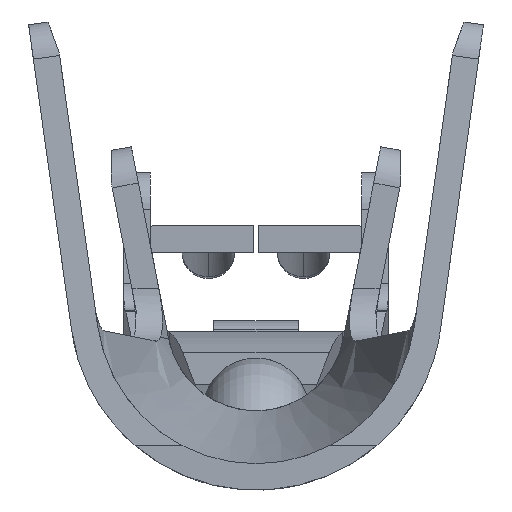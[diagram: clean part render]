
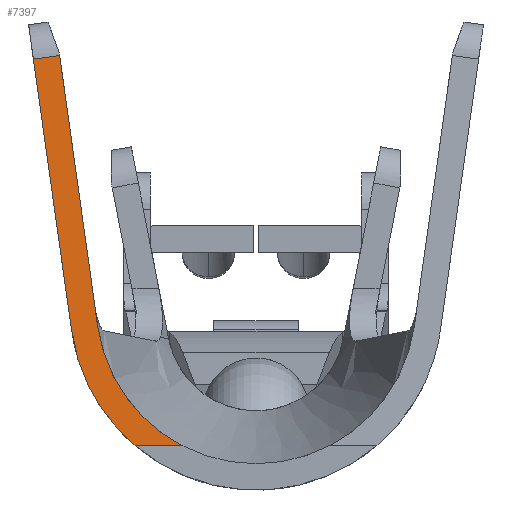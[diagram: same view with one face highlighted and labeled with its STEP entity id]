
A CAD part, front view. The second image highlights one B-rep face of the part: STEP entity #7397.
In plain terms, the highlighted planar face has unit normal (0, -0.998, 0.062).
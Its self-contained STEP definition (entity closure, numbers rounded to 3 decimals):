
#13 = VECTOR ( 'NONE', #1316, 1000. ) ;
#239 = DIRECTION ( 'NONE',  ( 0., -0.062, -0.998 ) ) ;
#319 = EDGE_CURVE ( 'NONE', #6120, #3955, #1105, .T. ) ;
#474 = CARTESIAN_POINT ( 'NONE',  ( -0.93, -4.743, -2.258 ) ) ;
#768 = VERTEX_POINT ( 'NONE', #2035 ) ;
#892 = ORIENTED_EDGE ( 'NONE', *, *, #319, .F. ) ;
#995 = VECTOR ( 'NONE', #4025, 1000. ) ;
#1105 = LINE ( 'NONE', #3718, #8045 ) ;
#1187 = LINE ( 'NONE', #8018, #995 ) ;
#1316 = DIRECTION ( 'NONE',  ( 0.99, 0.009, 0.139 ) ) ;
#1602 = VERTEX_POINT ( 'NONE', #4962 ) ;
#1620 = AXIS2_PLACEMENT_3D ( 'NONE', #6358, #3668, #239 ) ;
#1821 = CARTESIAN_POINT ( 'NONE',  ( -1.275, -4.723, -1.938 ) ) ;
#1880 = EDGE_CURVE ( 'NONE', #1602, #8000, #2816, .T. ) ;
#2035 = CARTESIAN_POINT ( 'NONE',  ( -1.497, -4.68, -1.248 ) ) ;
#2176 = PLANE ( 'NONE',  #1620 ) ;
#2337 = EDGE_CURVE ( 'NONE', #1602, #7081, #8230, .T. ) ;
#2407 = CARTESIAN_POINT ( 'NONE',  ( -1.857, -4.52, 1.31 ) ) ;
#2603 = CARTESIAN_POINT ( 'NONE',  ( -1.144, -4.75, -2.378 ) ) ;
#2770 = CARTESIAN_POINT ( 'NONE',  ( -2.104, -4.522, 1.275 ) ) ;
#2798 = ORIENTED_EDGE ( 'NONE', *, *, #5814, .F. ) ;
#2816 = LINE ( 'NONE', #2770, #4200 ) ;
#2915 = ORIENTED_EDGE ( 'NONE', *, *, #1880, .T. ) ;
#3623 = FACE_OUTER_BOUND ( 'NONE', #8695, .T. ) ;
#3668 = DIRECTION ( 'NONE',  ( 0., 0.998, -0.062 ) ) ;
#3718 = CARTESIAN_POINT ( 'NONE',  ( -0.7, -4.75, -2.378 ) ) ;
#3859 = B_SPLINE_CURVE_WITH_KNOTS ( 'NONE', 3,
 ( #4632, #5976, #8713, #6027, #2603 ),
 .UNSPECIFIED., .F., .F.,
 ( 4, 1, 4 ),
 ( 0., 0.5, 1. ),
 .UNSPECIFIED. ) ;
#3955 = VERTEX_POINT ( 'NONE', #8400 ) ;
#4025 = DIRECTION ( 'NONE',  ( -0.139, 0.062, 0.988 ) ) ;
#4146 = CARTESIAN_POINT ( 'NONE',  ( -2.104, -4.522, 1.275 ) ) ;
#4200 = VECTOR ( 'NONE', #5363, 1000. ) ;
#4632 = CARTESIAN_POINT ( 'NONE',  ( -1.745, -4.682, -1.283 ) ) ;
#4633 = EDGE_CURVE ( 'NONE', #768, #7081, #1187, .T. ) ;
#4962 = CARTESIAN_POINT ( 'NONE',  ( -2.104, -4.522, 1.275 ) ) ;
#5263 = B_SPLINE_CURVE_WITH_KNOTS ( 'NONE', 3,
 ( #5286, #7986, #1821, #474, #6507 ),
 .UNSPECIFIED., .F., .F.,
 ( 4, 1, 4 ),
 ( 0., 0.5, 1. ),
 .UNSPECIFIED. ) ;
#5286 = CARTESIAN_POINT ( 'NONE',  ( -1.497, -4.68, -1.248 ) ) ;
#5363 = DIRECTION ( 'NONE',  ( 0.139, -0.062, -0.988 ) ) ;
#5375 = ORIENTED_EDGE ( 'NONE', *, *, #4633, .T. ) ;
#5505 = CARTESIAN_POINT ( 'NONE',  ( -1.745, -4.682, -1.283 ) ) ;
#5814 = EDGE_CURVE ( 'NONE', #768, #6120, #5263, .T. ) ;
#5869 = CARTESIAN_POINT ( 'NONE',  ( -0.7, -4.75, -2.378 ) ) ;
#5870 = DIRECTION ( 'NONE',  ( -1., 0., 0. ) ) ;
#5976 = CARTESIAN_POINT ( 'NONE',  ( -1.714, -4.696, -1.504 ) ) ;
#6027 = CARTESIAN_POINT ( 'NONE',  ( -1.313, -4.741, -2.234 ) ) ;
#6120 = VERTEX_POINT ( 'NONE', #5869 ) ;
#6358 = CARTESIAN_POINT ( 'NONE',  ( 4.793, -4.5, 1.635 ) ) ;
#6414 = ORIENTED_EDGE ( 'NONE', *, *, #6486, .T. ) ;
#6486 = EDGE_CURVE ( 'NONE', #8000, #3955, #3859, .T. ) ;
#6507 = CARTESIAN_POINT ( 'NONE',  ( -0.7, -4.75, -2.378 ) ) ;
#6866 = ORIENTED_EDGE ( 'NONE', *, *, #2337, .F. ) ;
#7081 = VERTEX_POINT ( 'NONE', #2407 ) ;
#7397 = ADVANCED_FACE ( 'NONE', ( #3623 ), #2176, .F. ) ;
#7986 = CARTESIAN_POINT ( 'NONE',  ( -1.461, -4.696, -1.505 ) ) ;
#8000 = VERTEX_POINT ( 'NONE', #5505 ) ;
#8018 = CARTESIAN_POINT ( 'NONE',  ( -1.497, -4.68, -1.248 ) ) ;
#8045 = VECTOR ( 'NONE', #5870, 1000. ) ;
#8230 = LINE ( 'NONE', #4146, #13 ) ;
#8400 = CARTESIAN_POINT ( 'NONE',  ( -1.144, -4.75, -2.378 ) ) ;
#8695 = EDGE_LOOP ( 'NONE', ( #5375, #6866, #2915, #6414, #892, #2798 ) ) ;
#8713 = CARTESIAN_POINT ( 'NONE',  ( -1.576, -4.72, -1.903 ) ) ;
